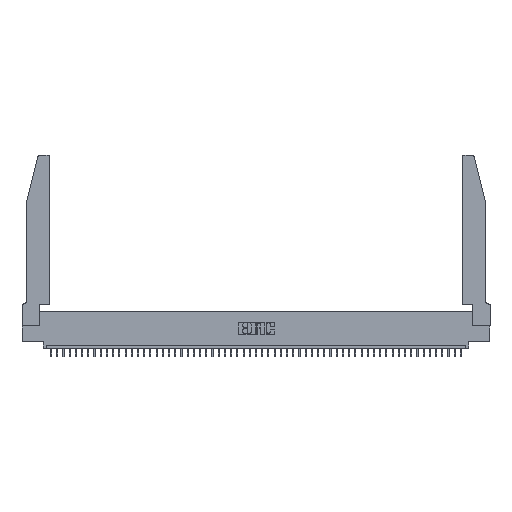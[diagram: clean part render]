
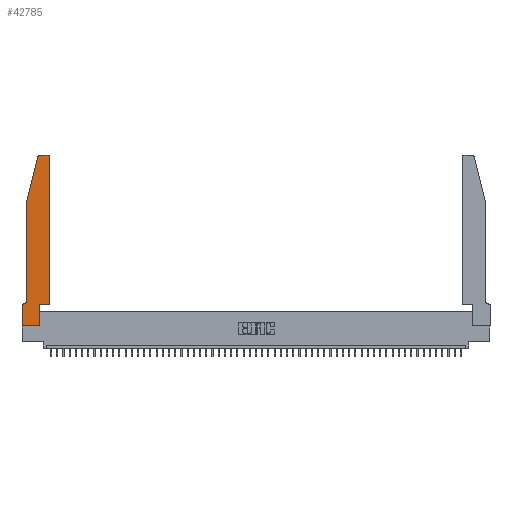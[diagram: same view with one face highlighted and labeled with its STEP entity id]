
A CAD part, top view. The second image highlights one B-rep face of the part: STEP entity #42785.
In plain terms, the highlighted planar face has unit normal (0, 0, 1).
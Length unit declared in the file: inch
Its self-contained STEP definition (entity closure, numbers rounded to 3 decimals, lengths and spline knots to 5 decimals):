
#1123 = ORIENTED_EDGE ( 'NONE', *, *, #44829, .T. ) ;
#1864 = FACE_OUTER_BOUND ( 'NONE', #23134, .T. ) ;
#2426 = VECTOR ( 'NONE', #47101, 39.37008 ) ;
#2562 = VERTEX_POINT ( 'NONE', #25328 ) ;
#4945 = EDGE_CURVE ( 'NONE', #36986, #8006, #27474, .T. ) ;
#5031 = DIRECTION ( 'NONE',  ( 0., 1., 0. ) ) ;
#5761 = VERTEX_POINT ( 'NONE', #38431 ) ;
#6245 = AXIS2_PLACEMENT_3D ( 'NONE', #10543, #42657, #38679 ) ;
#6339 = PLANE ( 'NONE',  #6245 ) ;
#6947 = CIRCLE ( 'NONE', #12805, 0.03 ) ;
#7147 = LINE ( 'NONE', #20025, #44116 ) ;
#7289 = CARTESIAN_POINT ( 'NONE',  ( 0.2865, 0., 0.37 ) ) ;
#7528 = ORIENTED_EDGE ( 'NONE', *, *, #42883, .T. ) ;
#7873 = CARTESIAN_POINT ( 'NONE',  ( 0., 0.35, 0.37 ) ) ;
#8006 = VERTEX_POINT ( 'NONE', #9067 ) ;
#8975 = LINE ( 'NONE', #41085, #18233 ) ;
#9067 = CARTESIAN_POINT ( 'NONE',  ( 0.0755, 0.42, 0.37 ) ) ;
#10543 = CARTESIAN_POINT ( 'NONE',  ( 0., 0.35, 0.37 ) ) ;
#10854 = DIRECTION ( 'NONE',  ( 1., 0., 0. ) ) ;
#11103 = LINE ( 'NONE', #51387, #26645 ) ;
#11238 = DIRECTION ( 'NONE',  ( 0., 0., 1. ) ) ;
#11277 = VERTEX_POINT ( 'NONE', #29297 ) ;
#12475 = DIRECTION ( 'NONE',  ( -1., 0., 0. ) ) ;
#12805 = AXIS2_PLACEMENT_3D ( 'NONE', #33454, #21089, #17659 ) ;
#13530 = CARTESIAN_POINT ( 'NONE',  ( 0.0055, 0.42, 0.37 ) ) ;
#14003 = EDGE_CURVE ( 'NONE', #11277, #20259, #48126, .T. ) ;
#14110 = DIRECTION ( 'NONE',  ( 0., -1., 0. ) ) ;
#14375 = VERTEX_POINT ( 'NONE', #40926 ) ;
#15004 = CARTESIAN_POINT ( 'NONE',  ( 0.4505, 0.35, 0.37 ) ) ;
#15628 = CARTESIAN_POINT ( 'NONE',  ( 0.0755, 2., 0.37 ) ) ;
#16450 = AXIS2_PLACEMENT_3D ( 'NONE', #18111, #11238, #27037 ) ;
#17293 = ORIENTED_EDGE ( 'NONE', *, *, #17614, .T. ) ;
#17583 = CARTESIAN_POINT ( 'NONE',  ( 0.0755, 2., 0.37 ) ) ;
#17614 = EDGE_CURVE ( 'NONE', #24115, #36255, #36847, .T. ) ;
#17659 = DIRECTION ( 'NONE',  ( 1., 0., 0. ) ) ;
#17752 = ORIENTED_EDGE ( 'NONE', *, *, #51028, .T. ) ;
#18111 = CARTESIAN_POINT ( 'NONE',  ( 0.284, 2.72, 0.37 ) ) ;
#18233 = VECTOR ( 'NONE', #5031, 39.37008 ) ;
#18555 = CARTESIAN_POINT ( 'NONE',  ( 0.4505, 0.35, 0.37 ) ) ;
#18750 = VECTOR ( 'NONE', #21796, 39.37008 ) ;
#20025 = CARTESIAN_POINT ( 'NONE',  ( 0., 0., 0.37 ) ) ;
#20259 = VERTEX_POINT ( 'NONE', #7873 ) ;
#21089 = DIRECTION ( 'NONE',  ( 0., 0., 1. ) ) ;
#21540 = LINE ( 'NONE', #17583, #18750 ) ;
#21796 = DIRECTION ( 'NONE',  ( -0.239, -0.971, 0. ) ) ;
#23134 = EDGE_LOOP ( 'NONE', ( #17293, #1123, #36929, #42033, #51236, #43204, #37557, #46948, #37737, #50230, #7528, #17752 ) ) ;
#23210 = DIRECTION ( 'NONE',  ( 1., 0., 0. ) ) ;
#23920 = LINE ( 'NONE', #15004, #30611 ) ;
#24115 = VERTEX_POINT ( 'NONE', #37713 ) ;
#24248 = EDGE_CURVE ( 'NONE', #41214, #49997, #7147, .T. ) ;
#25328 = CARTESIAN_POINT ( 'NONE',  ( 0.25487, 2.72718, 0.37 ) ) ;
#26645 = VECTOR ( 'NONE', #10854, 39.37008 ) ;
#27037 = DIRECTION ( 'NONE',  ( 1., 0., 0. ) ) ;
#27474 = LINE ( 'NONE', #15628, #45757 ) ;
#28061 = EDGE_CURVE ( 'NONE', #5761, #45241, #11103, .T. ) ;
#28242 = CIRCLE ( 'NONE', #16450, 0.03 ) ;
#28536 = EDGE_CURVE ( 'NONE', #49997, #5761, #8975, .T. ) ;
#28946 = DIRECTION ( 'NONE',  ( -1., 0., 0. ) ) ;
#29297 = CARTESIAN_POINT ( 'NONE',  ( 0.0055, 0.35, 0.37 ) ) ;
#29740 = CARTESIAN_POINT ( 'NONE',  ( 0.284, 2.75, 0.37 ) ) ;
#30611 = VECTOR ( 'NONE', #43435, 39.37008 ) ;
#31019 = EDGE_CURVE ( 'NONE', #8006, #11277, #48706, .T. ) ;
#32717 = CARTESIAN_POINT ( 'NONE',  ( 0.0755, 2., 0.37 ) ) ;
#32894 = CARTESIAN_POINT ( 'NONE',  ( 0.2605, 2.75, 0.37 ) ) ;
#33454 = CARTESIAN_POINT ( 'NONE',  ( 0.4205, 2.72, 0.37 ) ) ;
#33711 = VECTOR ( 'NONE', #28946, 39.37008 ) ;
#34097 = LINE ( 'NONE', #50185, #48446 ) ;
#35474 = CARTESIAN_POINT ( 'NONE',  ( 0.0755, 0.35, 0.37 ) ) ;
#36255 = VERTEX_POINT ( 'NONE', #29740 ) ;
#36847 = LINE ( 'NONE', #32894, #33711 ) ;
#36929 = ORIENTED_EDGE ( 'NONE', *, *, #41885, .T. ) ;
#36986 = VERTEX_POINT ( 'NONE', #32717 ) ;
#37209 = DIRECTION ( 'NONE',  ( 0., 0., -1. ) ) ;
#37557 = ORIENTED_EDGE ( 'NONE', *, *, #45161, .T. ) ;
#37713 = CARTESIAN_POINT ( 'NONE',  ( 0.4205, 2.75, 0.37 ) ) ;
#37737 = ORIENTED_EDGE ( 'NONE', *, *, #28536, .T. ) ;
#38431 = CARTESIAN_POINT ( 'NONE',  ( 0.2865, 0.35, 0.37 ) ) ;
#38679 = DIRECTION ( 'NONE',  ( 1., 0., 0. ) ) ;
#40926 = CARTESIAN_POINT ( 'NONE',  ( 0.4505, 2.72, 0.37 ) ) ;
#41085 = CARTESIAN_POINT ( 'NONE',  ( 0.2865, 0.35, 0.37 ) ) ;
#41214 = VERTEX_POINT ( 'NONE', #51376 ) ;
#41885 = EDGE_CURVE ( 'NONE', #2562, #36986, #21540, .T. ) ;
#42033 = ORIENTED_EDGE ( 'NONE', *, *, #4945, .T. ) ;
#42657 = DIRECTION ( 'NONE',  ( 0., 0., 1. ) ) ;
#42785 = ADVANCED_FACE ( 'NONE', ( #1864 ), #6339, .T. ) ;
#42883 = EDGE_CURVE ( 'NONE', #45241, #14375, #23920, .T. ) ;
#43023 = DIRECTION ( 'NONE',  ( 0., -1., 0. ) ) ;
#43204 = ORIENTED_EDGE ( 'NONE', *, *, #14003, .T. ) ;
#43435 = DIRECTION ( 'NONE',  ( 0., 1., 0. ) ) ;
#44116 = VECTOR ( 'NONE', #23210, 39.37008 ) ;
#44829 = EDGE_CURVE ( 'NONE', #36255, #2562, #28242, .T. ) ;
#45161 = EDGE_CURVE ( 'NONE', #20259, #41214, #34097, .T. ) ;
#45241 = VERTEX_POINT ( 'NONE', #18555 ) ;
#45757 = VECTOR ( 'NONE', #43023, 39.37008 ) ;
#46948 = ORIENTED_EDGE ( 'NONE', *, *, #24248, .T. ) ;
#47101 = DIRECTION ( 'NONE',  ( -1., 0., 0. ) ) ;
#48126 = LINE ( 'NONE', #35474, #2426 ) ;
#48446 = VECTOR ( 'NONE', #14110, 39.37008 ) ;
#48706 = CIRCLE ( 'NONE', #51219, 0.07 ) ;
#49997 = VERTEX_POINT ( 'NONE', #7289 ) ;
#50185 = CARTESIAN_POINT ( 'NONE',  ( 0., 0., 0.37 ) ) ;
#50230 = ORIENTED_EDGE ( 'NONE', *, *, #28061, .T. ) ;
#51028 = EDGE_CURVE ( 'NONE', #14375, #24115, #6947, .T. ) ;
#51219 = AXIS2_PLACEMENT_3D ( 'NONE', #13530, #37209, #12475 ) ;
#51236 = ORIENTED_EDGE ( 'NONE', *, *, #31019, .T. ) ;
#51376 = CARTESIAN_POINT ( 'NONE',  ( 0., 0., 0.37 ) ) ;
#51387 = CARTESIAN_POINT ( 'NONE',  ( 0.4505, 0.35, 0.37 ) ) ;
